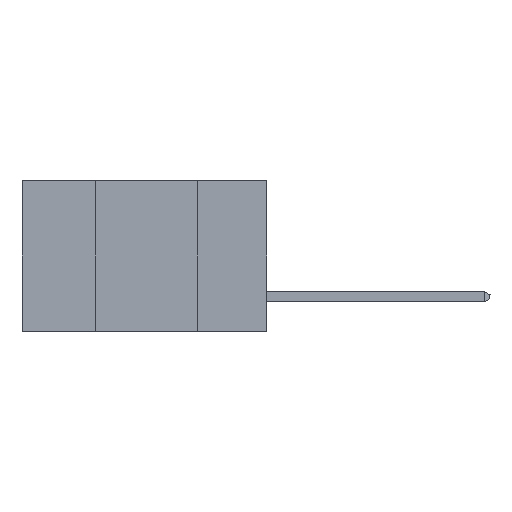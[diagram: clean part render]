
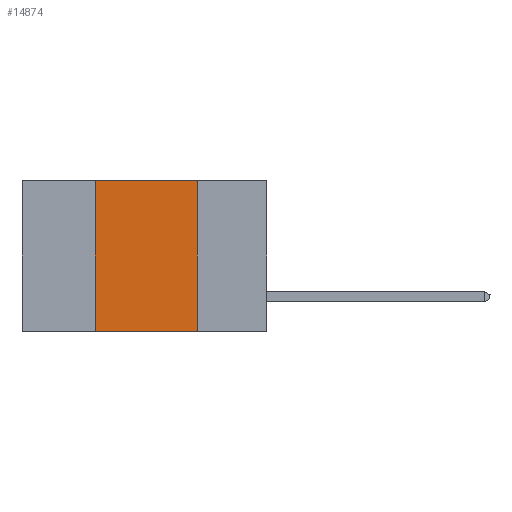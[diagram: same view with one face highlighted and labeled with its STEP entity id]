
A CAD part, left-side view. The second image highlights one B-rep face of the part: STEP entity #14874.
In plain terms, the highlighted planar face has unit normal (-1, 0, 0).
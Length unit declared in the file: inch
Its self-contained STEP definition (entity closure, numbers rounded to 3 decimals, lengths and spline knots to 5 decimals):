
#843 = LINE ( 'NONE', #7316, #25884 ) ;
#954 = EDGE_LOOP ( 'NONE', ( #26810, #12242, #14464, #25192 ) ) ;
#1263 = VERTEX_POINT ( 'NONE', #4944 ) ;
#1787 = DIRECTION ( 'NONE',  ( 0., 0., 1. ) ) ;
#3701 = CARTESIAN_POINT ( 'NONE',  ( 0., 0.42, -0.37 ) ) ;
#4944 = CARTESIAN_POINT ( 'NONE',  ( 0., 0.42, 0. ) ) ;
#6033 = VERTEX_POINT ( 'NONE', #24791 ) ;
#7316 = CARTESIAN_POINT ( 'NONE',  ( 0., 0.6, -0.37 ) ) ;
#7378 = CARTESIAN_POINT ( 'NONE',  ( 0., 0.6, 0. ) ) ;
#7647 = LINE ( 'NONE', #7378, #16967 ) ;
#7988 = CARTESIAN_POINT ( 'NONE',  ( 0., 0.42, 0. ) ) ;
#8875 = CARTESIAN_POINT ( 'NONE',  ( 0., 0.6, 0. ) ) ;
#9768 = EDGE_CURVE ( 'NONE', #20457, #6033, #10496, .T. ) ;
#10496 = LINE ( 'NONE', #25996, #18474 ) ;
#11433 = AXIS2_PLACEMENT_3D ( 'NONE', #8875, #21981, #26204 ) ;
#12242 = ORIENTED_EDGE ( 'NONE', *, *, #18410, .F. ) ;
#13390 = PLANE ( 'NONE',  #11433 ) ;
#14464 = ORIENTED_EDGE ( 'NONE', *, *, #15082, .F. ) ;
#14874 = ADVANCED_FACE ( 'NONE', ( #17614 ), #13390, .F. ) ;
#15082 = EDGE_CURVE ( 'NONE', #27422, #1263, #21110, .T. ) ;
#15536 = CARTESIAN_POINT ( 'NONE',  ( 0., 0.17, 0. ) ) ;
#16967 = VECTOR ( 'NONE', #22459, 39.37008 ) ;
#17262 = DIRECTION ( 'NONE',  ( 0., 0., -1. ) ) ;
#17614 = FACE_OUTER_BOUND ( 'NONE', #954, .T. ) ;
#18410 = EDGE_CURVE ( 'NONE', #1263, #20457, #7647, .T. ) ;
#18474 = VECTOR ( 'NONE', #17262, 39.37008 ) ;
#20457 = VERTEX_POINT ( 'NONE', #15536 ) ;
#21110 = LINE ( 'NONE', #7988, #24473 ) ;
#21981 = DIRECTION ( 'NONE',  ( 1., 0., 0. ) ) ;
#22459 = DIRECTION ( 'NONE',  ( 0., -1., 0. ) ) ;
#22807 = DIRECTION ( 'NONE',  ( 0., -1., 0. ) ) ;
#24473 = VECTOR ( 'NONE', #1787, 39.37008 ) ;
#24791 = CARTESIAN_POINT ( 'NONE',  ( 0., 0.17, -0.37 ) ) ;
#25192 = ORIENTED_EDGE ( 'NONE', *, *, #26215, .T. ) ;
#25884 = VECTOR ( 'NONE', #22807, 39.37008 ) ;
#25996 = CARTESIAN_POINT ( 'NONE',  ( 0., 0.17, 0. ) ) ;
#26204 = DIRECTION ( 'NONE',  ( 0., 0., -1. ) ) ;
#26215 = EDGE_CURVE ( 'NONE', #27422, #6033, #843, .T. ) ;
#26810 = ORIENTED_EDGE ( 'NONE', *, *, #9768, .F. ) ;
#27422 = VERTEX_POINT ( 'NONE', #3701 ) ;
